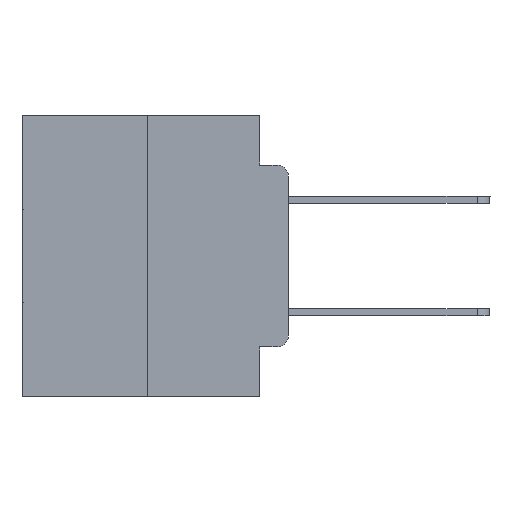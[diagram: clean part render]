
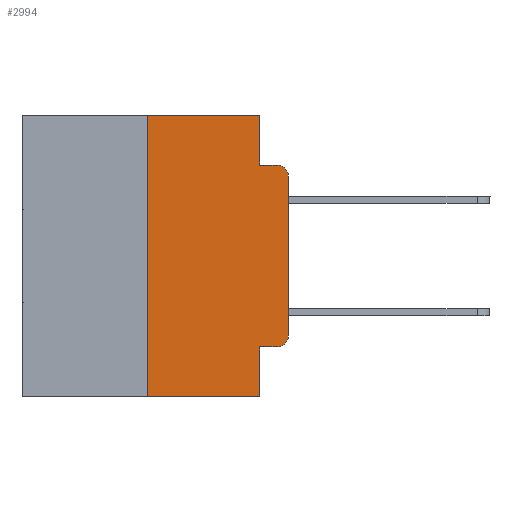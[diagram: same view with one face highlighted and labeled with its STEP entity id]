
A CAD part, left-side view. The second image highlights one B-rep face of the part: STEP entity #2994.
In plain terms, the highlighted planar face has unit normal (-1, 0, 0).
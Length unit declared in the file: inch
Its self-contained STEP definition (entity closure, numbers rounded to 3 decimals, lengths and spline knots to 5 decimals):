
#401 = CARTESIAN_POINT ( 'NONE',  ( 0., 0.25, -0.5 ) ) ;
#506 = ORIENTED_EDGE ( 'NONE', *, *, #15920, .F. ) ;
#633 = CARTESIAN_POINT ( 'NONE',  ( 0., 0.02, -0.0885 ) ) ;
#835 = VECTOR ( 'NONE', #3981, 39.37008 ) ;
#868 = CARTESIAN_POINT ( 'NONE',  ( 0., 0.25, 0. ) ) ;
#1530 = CARTESIAN_POINT ( 'NONE',  ( 0., 0.051, 0. ) ) ;
#2994 = ADVANCED_FACE ( 'NONE', ( #7011 ), #16079, .F. ) ;
#3474 = ORIENTED_EDGE ( 'NONE', *, *, #13027, .T. ) ;
#3523 = VERTEX_POINT ( 'NONE', #21358 ) ;
#3704 = ORIENTED_EDGE ( 'NONE', *, *, #23042, .T. ) ;
#3981 = DIRECTION ( 'NONE',  ( 0., 0., 1. ) ) ;
#4832 = CARTESIAN_POINT ( 'NONE',  ( 0., 0.473, 0. ) ) ;
#4890 = VECTOR ( 'NONE', #19824, 39.37008 ) ;
#4917 = DIRECTION ( 'NONE',  ( 1., 0., 0. ) ) ;
#5063 = VECTOR ( 'NONE', #12264, 39.37008 ) ;
#5767 = CARTESIAN_POINT ( 'NONE',  ( 0., 0.25, 0. ) ) ;
#5782 = DIRECTION ( 'NONE',  ( -1., 0., 0. ) ) ;
#5929 = DIRECTION ( 'NONE',  ( 0., 0., -1. ) ) ;
#5932 = ORIENTED_EDGE ( 'NONE', *, *, #23860, .F. ) ;
#6034 = VECTOR ( 'NONE', #12410, 39.37008 ) ;
#6142 = AXIS2_PLACEMENT_3D ( 'NONE', #13677, #13386, #8619 ) ;
#6380 = DIRECTION ( 'NONE',  ( 0., -1., 0. ) ) ;
#6402 = EDGE_CURVE ( 'NONE', #12066, #10883, #11074, .T. ) ;
#6666 = VERTEX_POINT ( 'NONE', #633 ) ;
#7011 = FACE_OUTER_BOUND ( 'NONE', #26680, .T. ) ;
#8431 = VERTEX_POINT ( 'NONE', #868 ) ;
#8619 = DIRECTION ( 'NONE',  ( 0., 0., -1. ) ) ;
#9439 = DIRECTION ( 'NONE',  ( 0., -1., 0. ) ) ;
#9569 = ORIENTED_EDGE ( 'NONE', *, *, #13388, .T. ) ;
#9722 = ORIENTED_EDGE ( 'NONE', *, *, #24817, .F. ) ;
#9919 = CIRCLE ( 'NONE', #6142, 0.02 ) ;
#10883 = VERTEX_POINT ( 'NONE', #17456 ) ;
#11074 = LINE ( 'NONE', #15689, #25331 ) ;
#11763 = CARTESIAN_POINT ( 'NONE',  ( 0., 0.051, 0. ) ) ;
#11812 = LINE ( 'NONE', #4832, #16081 ) ;
#12066 = VERTEX_POINT ( 'NONE', #401 ) ;
#12264 = DIRECTION ( 'NONE',  ( 0., 0., 1. ) ) ;
#12410 = DIRECTION ( 'NONE',  ( 0., -1., 0. ) ) ;
#12468 = ORIENTED_EDGE ( 'NONE', *, *, #6402, .T. ) ;
#12709 = VERTEX_POINT ( 'NONE', #11763 ) ;
#13027 = EDGE_CURVE ( 'NONE', #17535, #6666, #9919, .T. ) ;
#13386 = DIRECTION ( 'NONE',  ( -1., 0., 0. ) ) ;
#13388 = EDGE_CURVE ( 'NONE', #15928, #3523, #28901, .T. ) ;
#13677 = CARTESIAN_POINT ( 'NONE',  ( 0., 0.02, -0.1085 ) ) ;
#14006 = LINE ( 'NONE', #20827, #21362 ) ;
#14345 = LINE ( 'NONE', #21166, #6034 ) ;
#14500 = CARTESIAN_POINT ( 'NONE',  ( 0., 0., 0. ) ) ;
#15498 = VECTOR ( 'NONE', #6380, 39.37008 ) ;
#15689 = CARTESIAN_POINT ( 'NONE',  ( 0., 0.473, -0.5 ) ) ;
#15920 = EDGE_CURVE ( 'NONE', #17424, #10883, #14006, .T. ) ;
#15928 = VERTEX_POINT ( 'NONE', #19357 ) ;
#16079 = PLANE ( 'NONE',  #27616 ) ;
#16081 = VECTOR ( 'NONE', #9439, 39.37008 ) ;
#16557 = CARTESIAN_POINT ( 'NONE',  ( 0., 0.051, -0.0885 ) ) ;
#17224 = CARTESIAN_POINT ( 'NONE',  ( 0., 0.02, -0.3915 ) ) ;
#17424 = VERTEX_POINT ( 'NONE', #18276 ) ;
#17456 = CARTESIAN_POINT ( 'NONE',  ( 0., 0.051, -0.5 ) ) ;
#17535 = VERTEX_POINT ( 'NONE', #25650 ) ;
#18276 = CARTESIAN_POINT ( 'NONE',  ( 0., 0.051, -0.4115 ) ) ;
#18361 = ORIENTED_EDGE ( 'NONE', *, *, #25613, .F. ) ;
#18646 = EDGE_CURVE ( 'NONE', #12709, #19725, #21888, .T. ) ;
#19320 = ORIENTED_EDGE ( 'NONE', *, *, #18646, .F. ) ;
#19357 = CARTESIAN_POINT ( 'NONE',  ( 0., 0.02, -0.4115 ) ) ;
#19725 = VERTEX_POINT ( 'NONE', #16557 ) ;
#19824 = DIRECTION ( 'NONE',  ( 0., 0., -1. ) ) ;
#20136 = DIRECTION ( 'NONE',  ( 0., -1., 0. ) ) ;
#20827 = CARTESIAN_POINT ( 'NONE',  ( 0., 0.051, 0. ) ) ;
#21166 = CARTESIAN_POINT ( 'NONE',  ( 0., 0.051, -0.0885 ) ) ;
#21358 = CARTESIAN_POINT ( 'NONE',  ( 0., 0., -0.3915 ) ) ;
#21362 = VECTOR ( 'NONE', #27634, 39.37008 ) ;
#21888 = LINE ( 'NONE', #1530, #4890 ) ;
#21976 = ORIENTED_EDGE ( 'NONE', *, *, #23771, .T. ) ;
#22949 = LINE ( 'NONE', #14500, #5063 ) ;
#23042 = EDGE_CURVE ( 'NONE', #17424, #15928, #28369, .T. ) ;
#23771 = EDGE_CURVE ( 'NONE', #3523, #17535, #22949, .T. ) ;
#23860 = EDGE_CURVE ( 'NONE', #19725, #6666, #14345, .T. ) ;
#23911 = CARTESIAN_POINT ( 'NONE',  ( 0., 0.051, -0.4115 ) ) ;
#24817 = EDGE_CURVE ( 'NONE', #12066, #8431, #28336, .T. ) ;
#25108 = CARTESIAN_POINT ( 'NONE',  ( 0., 0.473, 0. ) ) ;
#25331 = VECTOR ( 'NONE', #20136, 39.37008 ) ;
#25613 = EDGE_CURVE ( 'NONE', #8431, #12709, #11812, .T. ) ;
#25650 = CARTESIAN_POINT ( 'NONE',  ( 0., 0., -0.1085 ) ) ;
#26528 = AXIS2_PLACEMENT_3D ( 'NONE', #17224, #5782, #5929 ) ;
#26680 = EDGE_LOOP ( 'NONE', ( #21976, #3474, #5932, #19320, #18361, #9722, #12468, #506, #3704, #9569 ) ) ;
#27616 = AXIS2_PLACEMENT_3D ( 'NONE', #25108, #4917, #28071 ) ;
#27634 = DIRECTION ( 'NONE',  ( 0., 0., -1. ) ) ;
#28071 = DIRECTION ( 'NONE',  ( 0., 0., -1. ) ) ;
#28336 = LINE ( 'NONE', #5767, #835 ) ;
#28369 = LINE ( 'NONE', #23911, #15498 ) ;
#28901 = CIRCLE ( 'NONE', #26528, 0.02 ) ;
